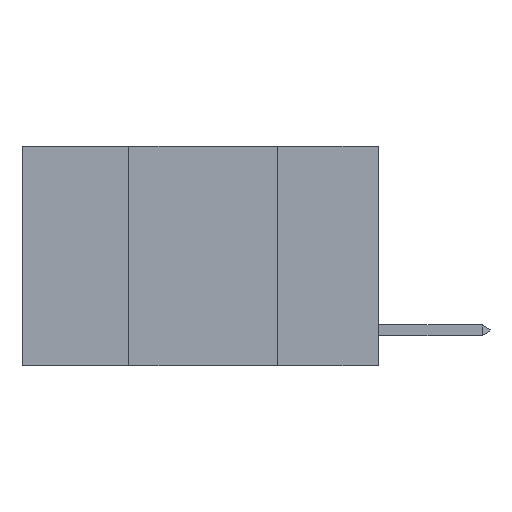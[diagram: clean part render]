
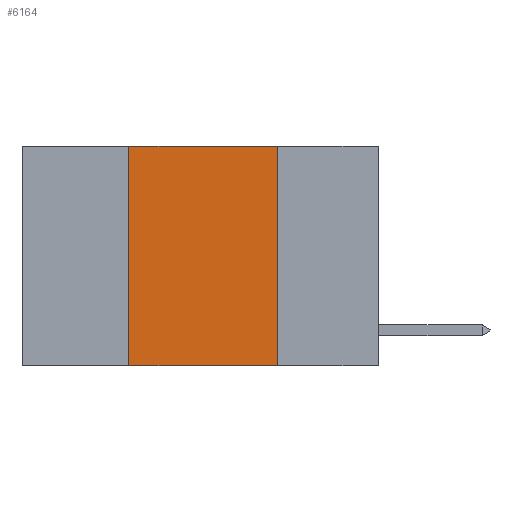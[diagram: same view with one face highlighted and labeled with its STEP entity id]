
A CAD part, left-side view. The second image highlights one B-rep face of the part: STEP entity #6164.
In plain terms, the highlighted planar face has unit normal (-1, 0, 0).
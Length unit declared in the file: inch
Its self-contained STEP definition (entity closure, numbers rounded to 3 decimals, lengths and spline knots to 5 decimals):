
#917 = LINE ( 'NONE', #4641, #12423 ) ;
#956 = CARTESIAN_POINT ( 'NONE',  ( 0., 0.42, 0. ) ) ;
#1199 = CARTESIAN_POINT ( 'NONE',  ( 0., 0.6, 0. ) ) ;
#1214 = VECTOR ( 'NONE', #13259, 39.37008 ) ;
#1335 = LINE ( 'NONE', #15836, #1214 ) ;
#2214 = DIRECTION ( 'NONE',  ( 0., -1., 0. ) ) ;
#2529 = FACE_OUTER_BOUND ( 'NONE', #8643, .T. ) ;
#2627 = DIRECTION ( 'NONE',  ( 0., -1., 0. ) ) ;
#3406 = ORIENTED_EDGE ( 'NONE', *, *, #6953, .F. ) ;
#4026 = AXIS2_PLACEMENT_3D ( 'NONE', #1199, #11736, #11822 ) ;
#4088 = CARTESIAN_POINT ( 'NONE',  ( 0., 0.6, 0. ) ) ;
#4205 = VERTEX_POINT ( 'NONE', #14689 ) ;
#4472 = VERTEX_POINT ( 'NONE', #7608 ) ;
#4641 = CARTESIAN_POINT ( 'NONE',  ( 0., 0.42, 0. ) ) ;
#5317 = EDGE_CURVE ( 'NONE', #10256, #4472, #1335, .T. ) ;
#6089 = VERTEX_POINT ( 'NONE', #956 ) ;
#6164 = ADVANCED_FACE ( 'NONE', ( #2529 ), #6656, .F. ) ;
#6415 = LINE ( 'NONE', #11666, #16357 ) ;
#6656 = PLANE ( 'NONE',  #4026 ) ;
#6953 = EDGE_CURVE ( 'NONE', #6089, #10256, #10552, .T. ) ;
#7409 = DIRECTION ( 'NONE',  ( 0., 0., 1. ) ) ;
#7608 = CARTESIAN_POINT ( 'NONE',  ( 0., 0.17, -0.37 ) ) ;
#8643 = EDGE_LOOP ( 'NONE', ( #14708, #3406, #10633, #16288 ) ) ;
#9280 = VECTOR ( 'NONE', #2627, 39.37008 ) ;
#10256 = VERTEX_POINT ( 'NONE', #13971 ) ;
#10552 = LINE ( 'NONE', #4088, #9280 ) ;
#10604 = EDGE_CURVE ( 'NONE', #4205, #6089, #917, .T. ) ;
#10633 = ORIENTED_EDGE ( 'NONE', *, *, #10604, .F. ) ;
#11666 = CARTESIAN_POINT ( 'NONE',  ( 0., 0.6, -0.37 ) ) ;
#11736 = DIRECTION ( 'NONE',  ( 1., 0., 0. ) ) ;
#11822 = DIRECTION ( 'NONE',  ( 0., 0., -1. ) ) ;
#12423 = VECTOR ( 'NONE', #7409, 39.37008 ) ;
#13116 = EDGE_CURVE ( 'NONE', #4205, #4472, #6415, .T. ) ;
#13259 = DIRECTION ( 'NONE',  ( 0., 0., -1. ) ) ;
#13971 = CARTESIAN_POINT ( 'NONE',  ( 0., 0.17, 0. ) ) ;
#14689 = CARTESIAN_POINT ( 'NONE',  ( 0., 0.42, -0.37 ) ) ;
#14708 = ORIENTED_EDGE ( 'NONE', *, *, #5317, .F. ) ;
#15836 = CARTESIAN_POINT ( 'NONE',  ( 0., 0.17, 0. ) ) ;
#16288 = ORIENTED_EDGE ( 'NONE', *, *, #13116, .T. ) ;
#16357 = VECTOR ( 'NONE', #2214, 39.37008 ) ;
